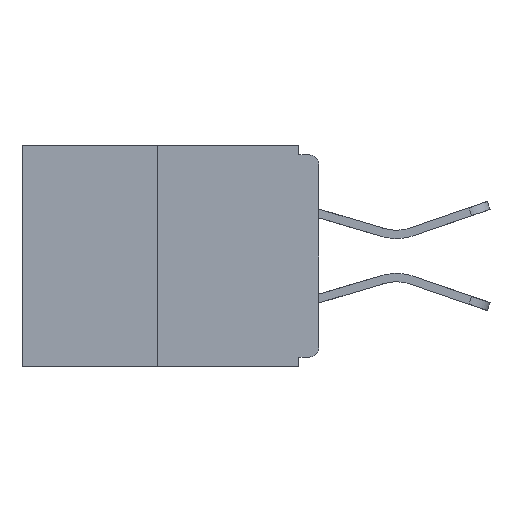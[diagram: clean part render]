
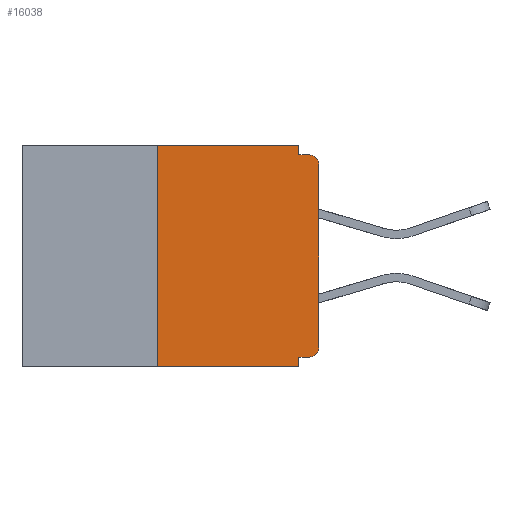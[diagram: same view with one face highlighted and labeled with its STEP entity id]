
A CAD part, left-side view. The second image highlights one B-rep face of the part: STEP entity #16038.
In plain terms, the highlighted planar face has unit normal (-1, 0, 0).
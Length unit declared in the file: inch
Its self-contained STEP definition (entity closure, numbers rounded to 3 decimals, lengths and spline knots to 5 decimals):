
#261 = VECTOR ( 'NONE', #14078, 39.37008 ) ;
#475 = VERTEX_POINT ( 'NONE', #8337 ) ;
#686 = ORIENTED_EDGE ( 'NONE', *, *, #4177, .F. ) ;
#1047 = DIRECTION ( 'NONE',  ( -1., 0., 0. ) ) ;
#1076 = CARTESIAN_POINT ( 'NONE',  ( 0., 0., -0.015 ) ) ;
#1372 = CARTESIAN_POINT ( 'NONE',  ( 0., 0.46, -0.343 ) ) ;
#1551 = CARTESIAN_POINT ( 'NONE',  ( 0., 0.25, 0. ) ) ;
#2061 = EDGE_CURVE ( 'NONE', #16445, #9504, #13944, .T. ) ;
#2078 = DIRECTION ( 'NONE',  ( -1., 0., 0. ) ) ;
#2275 = CARTESIAN_POINT ( 'NONE',  ( 0., 0.46, 0. ) ) ;
#2579 = EDGE_CURVE ( 'NONE', #13656, #7151, #8124, .T. ) ;
#2685 = AXIS2_PLACEMENT_3D ( 'NONE', #2275, #6073, #3635 ) ;
#3155 = CARTESIAN_POINT ( 'NONE',  ( 0., 0.031, -0.015 ) ) ;
#3230 = ORIENTED_EDGE ( 'NONE', *, *, #11842, .T. ) ;
#3525 = DIRECTION ( 'NONE',  ( 0., 0., -1. ) ) ;
#3617 = VERTEX_POINT ( 'NONE', #7301 ) ;
#3635 = DIRECTION ( 'NONE',  ( 0., 0., -1. ) ) ;
#3830 = CARTESIAN_POINT ( 'NONE',  ( 0., 0.015, -0.03 ) ) ;
#3998 = LINE ( 'NONE', #15622, #15922 ) ;
#4177 = EDGE_CURVE ( 'NONE', #13656, #12472, #8758, .T. ) ;
#4196 = VECTOR ( 'NONE', #10262, 39.37008 ) ;
#4275 = DIRECTION ( 'NONE',  ( 0., -1., 0. ) ) ;
#4593 = DIRECTION ( 'NONE',  ( 0., 0., 1. ) ) ;
#4896 = EDGE_CURVE ( 'NONE', #7398, #5540, #3998, .T. ) ;
#5540 = VERTEX_POINT ( 'NONE', #3155 ) ;
#5968 = CARTESIAN_POINT ( 'NONE',  ( 0., 0.015, -0.313 ) ) ;
#6012 = CARTESIAN_POINT ( 'NONE',  ( 0., 0.031, -0.328 ) ) ;
#6073 = DIRECTION ( 'NONE',  ( 1., 0., 0. ) ) ;
#6090 = EDGE_CURVE ( 'NONE', #9036, #7151, #14873, .T. ) ;
#6181 = PLANE ( 'NONE',  #2685 ) ;
#6269 = CARTESIAN_POINT ( 'NONE',  ( 0., 0.25, 0. ) ) ;
#6365 = VECTOR ( 'NONE', #15170, 39.37008 ) ;
#6381 = ORIENTED_EDGE ( 'NONE', *, *, #15111, .F. ) ;
#6427 = ORIENTED_EDGE ( 'NONE', *, *, #2061, .T. ) ;
#6780 = LINE ( 'NONE', #8059, #11147 ) ;
#7151 = VERTEX_POINT ( 'NONE', #13858 ) ;
#7301 = CARTESIAN_POINT ( 'NONE',  ( 0., 0., -0.03 ) ) ;
#7398 = VERTEX_POINT ( 'NONE', #9140 ) ;
#7973 = DIRECTION ( 'NONE',  ( 0., 0., -1. ) ) ;
#8059 = CARTESIAN_POINT ( 'NONE',  ( 0., 0.46, 0. ) ) ;
#8104 = ORIENTED_EDGE ( 'NONE', *, *, #10637, .F. ) ;
#8124 = LINE ( 'NONE', #1372, #4196 ) ;
#8278 = ORIENTED_EDGE ( 'NONE', *, *, #6090, .F. ) ;
#8337 = CARTESIAN_POINT ( 'NONE',  ( 0., 0.015, -0.015 ) ) ;
#8612 = ORIENTED_EDGE ( 'NONE', *, *, #12456, .T. ) ;
#8758 = LINE ( 'NONE', #6269, #13363 ) ;
#8826 = CARTESIAN_POINT ( 'NONE',  ( 0., 0.25, -0.343 ) ) ;
#8854 = EDGE_LOOP ( 'NONE', ( #13705, #686, #12321, #8278, #8104, #6427, #3230, #8612, #6381, #14042 ) ) ;
#9036 = VERTEX_POINT ( 'NONE', #6012 ) ;
#9140 = CARTESIAN_POINT ( 'NONE',  ( 0., 0.031, 0. ) ) ;
#9292 = FACE_OUTER_BOUND ( 'NONE', #8854, .T. ) ;
#9504 = VERTEX_POINT ( 'NONE', #13540 ) ;
#9874 = LINE ( 'NONE', #12883, #12481 ) ;
#10262 = DIRECTION ( 'NONE',  ( 0., -1., 0. ) ) ;
#10637 = EDGE_CURVE ( 'NONE', #16445, #9036, #9874, .T. ) ;
#11147 = VECTOR ( 'NONE', #4275, 39.37008 ) ;
#11346 = AXIS2_PLACEMENT_3D ( 'NONE', #5968, #2078, #3525 ) ;
#11422 = DIRECTION ( 'NONE',  ( 0., 0., -1. ) ) ;
#11842 = EDGE_CURVE ( 'NONE', #9504, #3617, #14404, .T. ) ;
#12321 = ORIENTED_EDGE ( 'NONE', *, *, #2579, .T. ) ;
#12456 = EDGE_CURVE ( 'NONE', #3617, #475, #14389, .T. ) ;
#12472 = VERTEX_POINT ( 'NONE', #1551 ) ;
#12481 = VECTOR ( 'NONE', #13885, 39.37008 ) ;
#12738 = AXIS2_PLACEMENT_3D ( 'NONE', #3830, #1047, #15245 ) ;
#12883 = CARTESIAN_POINT ( 'NONE',  ( 0., 0., -0.328 ) ) ;
#13363 = VECTOR ( 'NONE', #4593, 39.37008 ) ;
#13540 = CARTESIAN_POINT ( 'NONE',  ( 0., 0., -0.313 ) ) ;
#13656 = VERTEX_POINT ( 'NONE', #8826 ) ;
#13705 = ORIENTED_EDGE ( 'NONE', *, *, #14131, .F. ) ;
#13858 = CARTESIAN_POINT ( 'NONE',  ( 0., 0.031, -0.343 ) ) ;
#13869 = CARTESIAN_POINT ( 'NONE',  ( 0., 0.031, -0.343 ) ) ;
#13885 = DIRECTION ( 'NONE',  ( 0., 1., 0. ) ) ;
#13944 = CIRCLE ( 'NONE', #11346, 0.015 ) ;
#14042 = ORIENTED_EDGE ( 'NONE', *, *, #4896, .F. ) ;
#14078 = DIRECTION ( 'NONE',  ( 0., 0., 1. ) ) ;
#14131 = EDGE_CURVE ( 'NONE', #12472, #7398, #6780, .T. ) ;
#14389 = CIRCLE ( 'NONE', #12738, 0.015 ) ;
#14404 = LINE ( 'NONE', #15453, #261 ) ;
#14427 = CARTESIAN_POINT ( 'NONE',  ( 0., 0.015, -0.328 ) ) ;
#14873 = LINE ( 'NONE', #13869, #15871 ) ;
#15111 = EDGE_CURVE ( 'NONE', #5540, #475, #16308, .T. ) ;
#15170 = DIRECTION ( 'NONE',  ( 0., -1., 0. ) ) ;
#15245 = DIRECTION ( 'NONE',  ( 0., 0., -1. ) ) ;
#15453 = CARTESIAN_POINT ( 'NONE',  ( 0., 0., 0. ) ) ;
#15622 = CARTESIAN_POINT ( 'NONE',  ( 0., 0.031, 0. ) ) ;
#15871 = VECTOR ( 'NONE', #11422, 39.37008 ) ;
#15922 = VECTOR ( 'NONE', #7973, 39.37008 ) ;
#16038 = ADVANCED_FACE ( 'NONE', ( #9292 ), #6181, .F. ) ;
#16308 = LINE ( 'NONE', #1076, #6365 ) ;
#16445 = VERTEX_POINT ( 'NONE', #14427 ) ;
